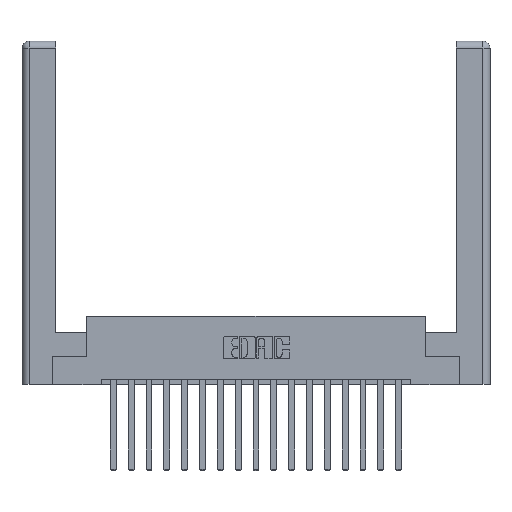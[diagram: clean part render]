
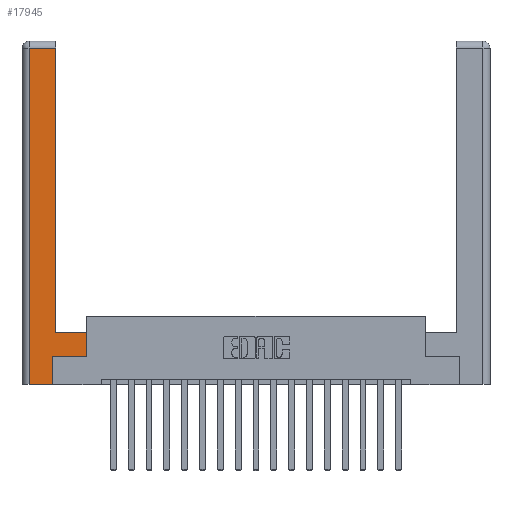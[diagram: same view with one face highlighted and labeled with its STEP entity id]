
A CAD part, top view. The second image highlights one B-rep face of the part: STEP entity #17945.
In plain terms, the highlighted planar face has unit normal (0, 0, 1).
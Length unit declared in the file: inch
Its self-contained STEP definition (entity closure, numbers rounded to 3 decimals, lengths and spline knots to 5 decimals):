
#98 = DIRECTION ( 'NONE',  ( 1., 0., 0. ) ) ;
#365 = LINE ( 'NONE', #6376, #16765 ) ;
#1136 = VECTOR ( 'NONE', #17911, 39.37008 ) ;
#1274 = CARTESIAN_POINT ( 'NONE',  ( 0.265, 0.245, 0. ) ) ;
#1291 = EDGE_CURVE ( 'NONE', #14571, #12017, #6128, .T. ) ;
#1540 = EDGE_CURVE ( 'NONE', #9829, #14345, #17314, .T. ) ;
#2180 = LINE ( 'NONE', #16886, #6504 ) ;
#2193 = CARTESIAN_POINT ( 'NONE',  ( 0.295, 2.94, 0. ) ) ;
#2265 = VECTOR ( 'NONE', #98, 39.37008 ) ;
#3235 = CARTESIAN_POINT ( 'NONE',  ( 0.565, 0.245, 0. ) ) ;
#3263 = CARTESIAN_POINT ( 'NONE',  ( 0.0615, 2.94, 0. ) ) ;
#4003 = AXIS2_PLACEMENT_3D ( 'NONE', #12998, #12811, #14272 ) ;
#4295 = ORIENTED_EDGE ( 'NONE', *, *, #5496, .T. ) ;
#4873 = ORIENTED_EDGE ( 'NONE', *, *, #1291, .T. ) ;
#5496 = EDGE_CURVE ( 'NONE', #14345, #14571, #14658, .T. ) ;
#5699 = CARTESIAN_POINT ( 'NONE',  ( 0.295, 0.45, 0. ) ) ;
#6128 = LINE ( 'NONE', #3263, #1136 ) ;
#6376 = CARTESIAN_POINT ( 'NONE',  ( 0.565, 0.45, 0. ) ) ;
#6386 = ORIENTED_EDGE ( 'NONE', *, *, #16843, .T. ) ;
#6395 = DIRECTION ( 'NONE',  ( 0., -1., 0. ) ) ;
#6406 = EDGE_CURVE ( 'NONE', #8217, #8763, #17343, .T. ) ;
#6504 = VECTOR ( 'NONE', #9691, 39.37008 ) ;
#6905 = LINE ( 'NONE', #13708, #18102 ) ;
#7403 = CARTESIAN_POINT ( 'NONE',  ( 0.0615, 2.94, 0. ) ) ;
#7484 = DIRECTION ( 'NONE',  ( 1., 0., 0. ) ) ;
#7852 = ORIENTED_EDGE ( 'NONE', *, *, #1540, .T. ) ;
#8166 = ORIENTED_EDGE ( 'NONE', *, *, #14486, .T. ) ;
#8217 = VERTEX_POINT ( 'NONE', #16063 ) ;
#8763 = VERTEX_POINT ( 'NONE', #9329 ) ;
#9004 = ORIENTED_EDGE ( 'NONE', *, *, #11523, .T. ) ;
#9329 = CARTESIAN_POINT ( 'NONE',  ( 0.265, 0., 0. ) ) ;
#9688 = EDGE_LOOP ( 'NONE', ( #4295, #4873, #8166, #10852, #13712, #9004, #6386, #7852 ) ) ;
#9691 = DIRECTION ( 'NONE',  ( 0., 1., 0. ) ) ;
#9813 = VERTEX_POINT ( 'NONE', #1274 ) ;
#9829 = VERTEX_POINT ( 'NONE', #18359 ) ;
#9922 = PLANE ( 'NONE',  #4003 ) ;
#10106 = DIRECTION ( 'NONE',  ( 0., 1., 0. ) ) ;
#10852 = ORIENTED_EDGE ( 'NONE', *, *, #6406, .T. ) ;
#11523 = EDGE_CURVE ( 'NONE', #9813, #11618, #15015, .T. ) ;
#11618 = VERTEX_POINT ( 'NONE', #13681 ) ;
#11687 = VECTOR ( 'NONE', #10106, 39.37008 ) ;
#12017 = VERTEX_POINT ( 'NONE', #7403 ) ;
#12102 = DIRECTION ( 'NONE',  ( 0., 1., 0. ) ) ;
#12293 = EDGE_CURVE ( 'NONE', #8763, #9813, #2180, .T. ) ;
#12811 = DIRECTION ( 'NONE',  ( 0., 0., -1. ) ) ;
#12998 = CARTESIAN_POINT ( 'NONE',  ( 0., 0., 0. ) ) ;
#13681 = CARTESIAN_POINT ( 'NONE',  ( 0.565, 0.245, 0. ) ) ;
#13708 = CARTESIAN_POINT ( 'NONE',  ( 0.0615, 0., 0. ) ) ;
#13712 = ORIENTED_EDGE ( 'NONE', *, *, #12293, .T. ) ;
#14272 = DIRECTION ( 'NONE',  ( -1., 0., 0. ) ) ;
#14345 = VERTEX_POINT ( 'NONE', #15725 ) ;
#14486 = EDGE_CURVE ( 'NONE', #12017, #8217, #6905, .T. ) ;
#14548 = DIRECTION ( 'NONE',  ( -1., 0., 0. ) ) ;
#14571 = VERTEX_POINT ( 'NONE', #2193 ) ;
#14658 = LINE ( 'NONE', #14958, #11687 ) ;
#14812 = CARTESIAN_POINT ( 'NONE',  ( 0.265, 0., 0. ) ) ;
#14958 = CARTESIAN_POINT ( 'NONE',  ( 0.295, 3., 0. ) ) ;
#15015 = LINE ( 'NONE', #3235, #17514 ) ;
#15725 = CARTESIAN_POINT ( 'NONE',  ( 0.295, 0.45, 0. ) ) ;
#16063 = CARTESIAN_POINT ( 'NONE',  ( 0.0615, 0., 0. ) ) ;
#16765 = VECTOR ( 'NONE', #12102, 39.37008 ) ;
#16834 = VECTOR ( 'NONE', #14548, 39.37008 ) ;
#16843 = EDGE_CURVE ( 'NONE', #11618, #9829, #365, .T. ) ;
#16886 = CARTESIAN_POINT ( 'NONE',  ( 0.265, 0.245, 0. ) ) ;
#17314 = LINE ( 'NONE', #5699, #16834 ) ;
#17343 = LINE ( 'NONE', #14812, #2265 ) ;
#17514 = VECTOR ( 'NONE', #7484, 39.37008 ) ;
#17646 = FACE_OUTER_BOUND ( 'NONE', #9688, .T. ) ;
#17911 = DIRECTION ( 'NONE',  ( -1., 0., 0. ) ) ;
#17945 = ADVANCED_FACE ( 'NONE', ( #17646 ), #9922, .F. ) ;
#18102 = VECTOR ( 'NONE', #6395, 39.37008 ) ;
#18359 = CARTESIAN_POINT ( 'NONE',  ( 0.565, 0.45, 0. ) ) ;
